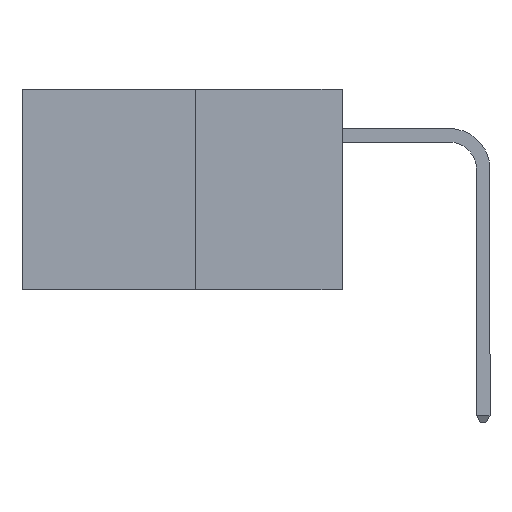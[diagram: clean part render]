
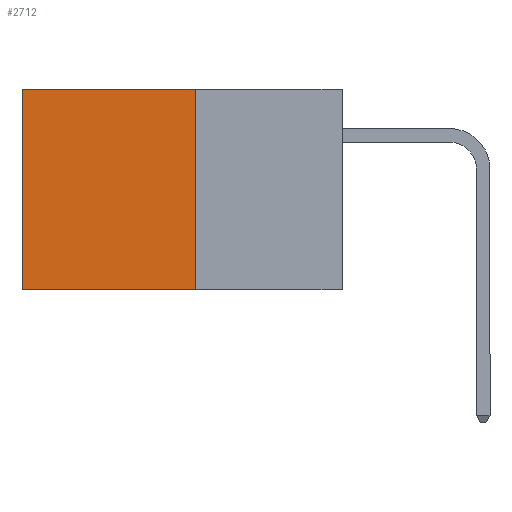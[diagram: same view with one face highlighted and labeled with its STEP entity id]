
A CAD part, left-side view. The second image highlights one B-rep face of the part: STEP entity #2712.
In plain terms, the highlighted planar face has unit normal (-1, 0, 0).
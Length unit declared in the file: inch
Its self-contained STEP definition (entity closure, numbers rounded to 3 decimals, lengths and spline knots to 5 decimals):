
#3 = ORIENTED_EDGE ( 'NONE', *, *, #6285, .T. ) ;
#84 = CARTESIAN_POINT ( 'NONE',  ( 0.277, 0.27, 0. ) ) ;
#146 = ORIENTED_EDGE ( 'NONE', *, *, #1549, .F. ) ;
#190 = ORIENTED_EDGE ( 'NONE', *, *, #8337, .F. ) ;
#376 = ORIENTED_EDGE ( 'NONE', *, *, #5320, .T. ) ;
#1012 = VECTOR ( 'NONE', #3248, 39.37008 ) ;
#1321 = CARTESIAN_POINT ( 'NONE',  ( 0.277, 0.59, 0. ) ) ;
#1440 = DIRECTION ( 'NONE',  ( 0., 0., -1. ) ) ;
#1549 = EDGE_CURVE ( 'NONE', #12761, #6444, #11182, .T. ) ;
#2005 = AXIS2_PLACEMENT_3D ( 'NONE', #4504, #4795, #1440 ) ;
#2712 = ADVANCED_FACE ( 'NONE', ( #10064 ), #12734, .F. ) ;
#2763 = CARTESIAN_POINT ( 'NONE',  ( 0.277, 0.59, -0.37 ) ) ;
#3248 = DIRECTION ( 'NONE',  ( 0., 1., 0. ) ) ;
#3540 = LINE ( 'NONE', #9115, #1012 ) ;
#4504 = CARTESIAN_POINT ( 'NONE',  ( 0.277, 0.27, -0.37 ) ) ;
#4795 = DIRECTION ( 'NONE',  ( 1., 0., 0. ) ) ;
#5320 = EDGE_CURVE ( 'NONE', #9046, #9531, #9894, .T. ) ;
#5664 = VECTOR ( 'NONE', #8412, 39.37008 ) ;
#6285 = EDGE_CURVE ( 'NONE', #12761, #9046, #3540, .T. ) ;
#6444 = VERTEX_POINT ( 'NONE', #12785 ) ;
#6822 = VECTOR ( 'NONE', #12794, 39.37008 ) ;
#7071 = VECTOR ( 'NONE', #13196, 39.37008 ) ;
#7505 = CARTESIAN_POINT ( 'NONE',  ( 0.277, 0.27, -0.37 ) ) ;
#8337 = EDGE_CURVE ( 'NONE', #6444, #9531, #9805, .T. ) ;
#8412 = DIRECTION ( 'NONE',  ( 0., 0., -1. ) ) ;
#9046 = VERTEX_POINT ( 'NONE', #1321 ) ;
#9115 = CARTESIAN_POINT ( 'NONE',  ( 0.277, 0.27, 0. ) ) ;
#9531 = VERTEX_POINT ( 'NONE', #11547 ) ;
#9805 = LINE ( 'NONE', #7505, #7071 ) ;
#9889 = EDGE_LOOP ( 'NONE', ( #376, #190, #146, #3 ) ) ;
#9894 = LINE ( 'NONE', #2763, #6822 ) ;
#10064 = FACE_OUTER_BOUND ( 'NONE', #9889, .T. ) ;
#10235 = CARTESIAN_POINT ( 'NONE',  ( 0.277, 0.27, -0.37 ) ) ;
#11182 = LINE ( 'NONE', #10235, #5664 ) ;
#11547 = CARTESIAN_POINT ( 'NONE',  ( 0.277, 0.59, -0.37 ) ) ;
#12734 = PLANE ( 'NONE',  #2005 ) ;
#12761 = VERTEX_POINT ( 'NONE', #84 ) ;
#12785 = CARTESIAN_POINT ( 'NONE',  ( 0.277, 0.27, -0.37 ) ) ;
#12794 = DIRECTION ( 'NONE',  ( 0., 0., -1. ) ) ;
#13196 = DIRECTION ( 'NONE',  ( 0., 1., 0. ) ) ;
